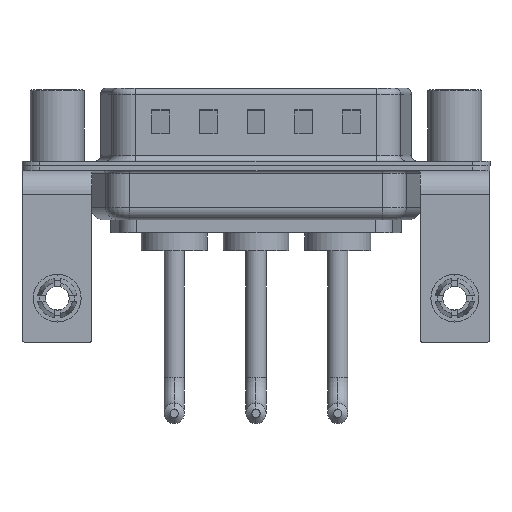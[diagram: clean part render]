
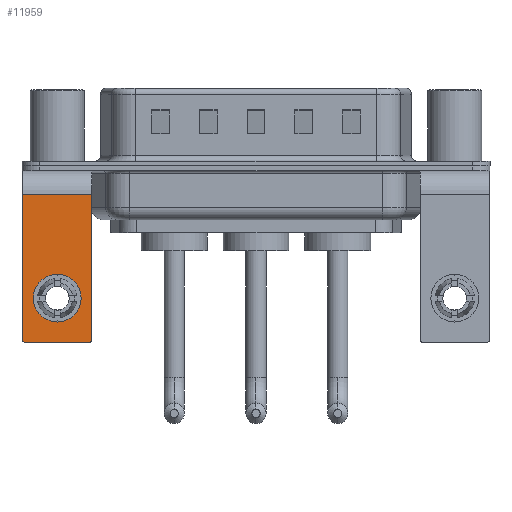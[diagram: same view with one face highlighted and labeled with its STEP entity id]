
A CAD part, front view. The second image highlights one B-rep face of the part: STEP entity #11959.
In plain terms, the highlighted planar face has unit normal (0, -1, 0).
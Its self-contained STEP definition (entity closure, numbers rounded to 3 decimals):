
#63 = CARTESIAN_POINT ( 'NONE',  ( -2.9, -6.25, -14.55 ) ) ;
#1056 = ORIENTED_EDGE ( 'NONE', *, *, #9136, .T. ) ;
#1064 = DIRECTION ( 'NONE',  ( 0., 0., -1. ) ) ;
#1823 = VERTEX_POINT ( 'NONE', #5602 ) ;
#2591 = CARTESIAN_POINT ( 'NONE',  ( 0., -6.25, -13.07 ) ) ;
#2992 = CARTESIAN_POINT ( 'NONE',  ( 0., -6.25, -9.07 ) ) ;
#2994 = EDGE_CURVE ( 'NONE', #1823, #10817, #14287, .T. ) ;
#3014 = CARTESIAN_POINT ( 'NONE',  ( 2.9, -6.25, -14.55 ) ) ;
#3553 = AXIS2_PLACEMENT_3D ( 'NONE', #14173, #9504, #13890 ) ;
#3733 = AXIS2_PLACEMENT_3D ( 'NONE', #5045, #17106, #9521 ) ;
#4156 = LINE ( 'NONE', #15824, #18837 ) ;
#4374 = VERTEX_POINT ( 'NONE', #9350 ) ;
#5045 = CARTESIAN_POINT ( 'NONE',  ( -2.65, -6.25, -14.55 ) ) ;
#5449 = VERTEX_POINT ( 'NONE', #2591 ) ;
#5602 = CARTESIAN_POINT ( 'NONE',  ( 2.9, -6.25, -2.4 ) ) ;
#6000 = EDGE_CURVE ( 'NONE', #16006, #13937, #6839, .T. ) ;
#6182 = ORIENTED_EDGE ( 'NONE', *, *, #17337, .T. ) ;
#6720 = EDGE_LOOP ( 'NONE', ( #17210, #6182 ) ) ;
#6839 = LINE ( 'NONE', #12583, #16416 ) ;
#7018 = VERTEX_POINT ( 'NONE', #63 ) ;
#7624 = LINE ( 'NONE', #15227, #19090 ) ;
#7921 = CIRCLE ( 'NONE', #18811, 2. ) ;
#8021 = CARTESIAN_POINT ( 'NONE',  ( -2.65, -6.25, -14.8 ) ) ;
#8292 = ORIENTED_EDGE ( 'NONE', *, *, #15608, .T. ) ;
#8795 = CIRCLE ( 'NONE', #10684, 0.25 ) ;
#8821 = CIRCLE ( 'NONE', #3553, 2. ) ;
#9136 = EDGE_CURVE ( 'NONE', #7018, #13937, #11830, .T. ) ;
#9350 = CARTESIAN_POINT ( 'NONE',  ( -2.9, -6.25, -2.4 ) ) ;
#9438 = ORIENTED_EDGE ( 'NONE', *, *, #18286, .T. ) ;
#9504 = DIRECTION ( 'NONE',  ( 0., 1., 0. ) ) ;
#9521 = DIRECTION ( 'NONE',  ( 0., 0., 1. ) ) ;
#10519 = DIRECTION ( 'NONE',  ( 0., 0., 1. ) ) ;
#10569 = DIRECTION ( 'NONE',  ( -1., 0., 0. ) ) ;
#10684 = AXIS2_PLACEMENT_3D ( 'NONE', #13433, #10704, #10519 ) ;
#10704 = DIRECTION ( 'NONE',  ( 0., -1., 0. ) ) ;
#10817 = VERTEX_POINT ( 'NONE', #3014 ) ;
#11113 = FACE_BOUND ( 'NONE', #6720, .T. ) ;
#11199 = VERTEX_POINT ( 'NONE', #2992 ) ;
#11406 = EDGE_LOOP ( 'NONE', ( #9438, #1056, #14006, #16739, #19154, #8292 ) ) ;
#11830 = CIRCLE ( 'NONE', #3733, 0.25 ) ;
#11959 = ADVANCED_FACE ( 'NONE', ( #11113, #15578 ), #12660, .F. ) ;
#12583 = CARTESIAN_POINT ( 'NONE',  ( 2.9, -6.25, -14.8 ) ) ;
#12660 = PLANE ( 'NONE',  #15912 ) ;
#13433 = CARTESIAN_POINT ( 'NONE',  ( 2.65, -6.25, -14.55 ) ) ;
#13890 = DIRECTION ( 'NONE',  ( 0., 0., 1. ) ) ;
#13937 = VERTEX_POINT ( 'NONE', #8021 ) ;
#14006 = ORIENTED_EDGE ( 'NONE', *, *, #6000, .F. ) ;
#14041 = CARTESIAN_POINT ( 'NONE',  ( 2.65, -6.25, -14.8 ) ) ;
#14173 = CARTESIAN_POINT ( 'NONE',  ( 0., -6.25, -11.07 ) ) ;
#14287 = LINE ( 'NONE', #15920, #16953 ) ;
#14787 = EDGE_CURVE ( 'NONE', #16006, #10817, #8795, .T. ) ;
#15227 = CARTESIAN_POINT ( 'NONE',  ( 2.9, -6.25, -2.4 ) ) ;
#15578 = FACE_OUTER_BOUND ( 'NONE', #11406, .T. ) ;
#15608 = EDGE_CURVE ( 'NONE', #1823, #4374, #7624, .T. ) ;
#15652 = DIRECTION ( 'NONE',  ( 0., 0., 1. ) ) ;
#15746 = EDGE_CURVE ( 'NONE', #5449, #11199, #8821, .T. ) ;
#15824 = CARTESIAN_POINT ( 'NONE',  ( -2.9, -6.25, -2.4 ) ) ;
#15912 = AXIS2_PLACEMENT_3D ( 'NONE', #18599, #17039, #17137 ) ;
#15920 = CARTESIAN_POINT ( 'NONE',  ( 2.9, -6.25, -2.4 ) ) ;
#16006 = VERTEX_POINT ( 'NONE', #14041 ) ;
#16416 = VECTOR ( 'NONE', #18906, 1000. ) ;
#16739 = ORIENTED_EDGE ( 'NONE', *, *, #14787, .T. ) ;
#16953 = VECTOR ( 'NONE', #1064, 1000. ) ;
#17039 = DIRECTION ( 'NONE',  ( 0., 1., 0. ) ) ;
#17106 = DIRECTION ( 'NONE',  ( 0., -1., 0. ) ) ;
#17137 = DIRECTION ( 'NONE',  ( 0., 0., 1. ) ) ;
#17210 = ORIENTED_EDGE ( 'NONE', *, *, #15746, .T. ) ;
#17290 = DIRECTION ( 'NONE',  ( 0., 0., -1. ) ) ;
#17337 = EDGE_CURVE ( 'NONE', #11199, #5449, #7921, .T. ) ;
#18286 = EDGE_CURVE ( 'NONE', #4374, #7018, #4156, .T. ) ;
#18585 = DIRECTION ( 'NONE',  ( 0., 1., 0. ) ) ;
#18599 = CARTESIAN_POINT ( 'NONE',  ( 2.9, -6.25, -2.4 ) ) ;
#18673 = CARTESIAN_POINT ( 'NONE',  ( 0., -6.25, -11.07 ) ) ;
#18811 = AXIS2_PLACEMENT_3D ( 'NONE', #18673, #18585, #15652 ) ;
#18837 = VECTOR ( 'NONE', #17290, 1000. ) ;
#18906 = DIRECTION ( 'NONE',  ( -1., 0., 0. ) ) ;
#19090 = VECTOR ( 'NONE', #10569, 1000. ) ;
#19154 = ORIENTED_EDGE ( 'NONE', *, *, #2994, .F. ) ;
